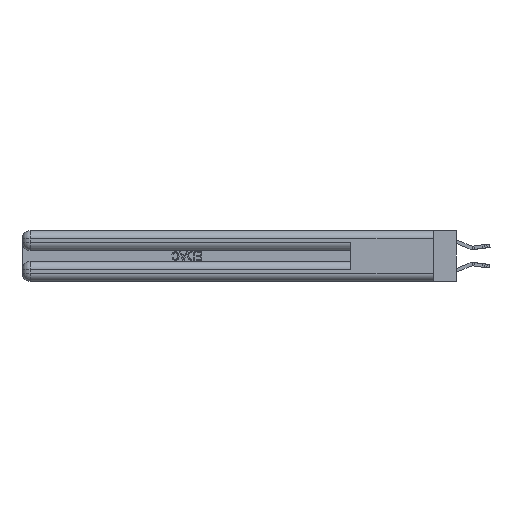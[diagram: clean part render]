
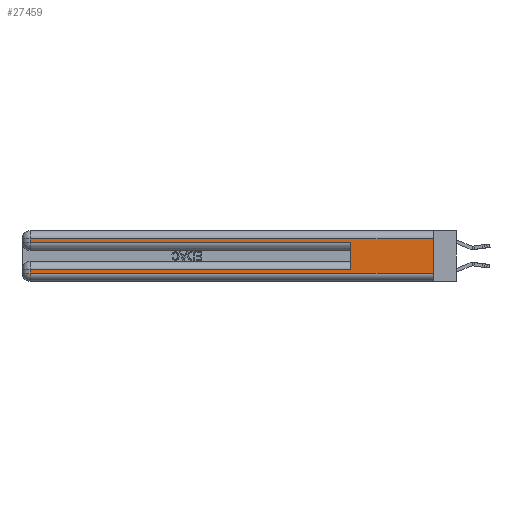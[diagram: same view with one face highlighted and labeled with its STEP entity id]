
A CAD part, left-side view. The second image highlights one B-rep face of the part: STEP entity #27459.
In plain terms, the highlighted planar face has unit normal (-1, 0, 0).
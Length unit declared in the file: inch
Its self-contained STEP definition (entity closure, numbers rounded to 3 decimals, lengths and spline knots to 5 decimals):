
#120 = CARTESIAN_POINT ( 'NONE',  ( 0., 0., 0.31 ) ) ;
#1399 = ORIENTED_EDGE ( 'NONE', *, *, #13065, .F. ) ;
#3127 = ORIENTED_EDGE ( 'NONE', *, *, #30233, .T. ) ;
#3662 = CARTESIAN_POINT ( 'NONE',  ( 0., 2.94, 0.06 ) ) ;
#4839 = VECTOR ( 'NONE', #20133, 39.37008 ) ;
#5645 = DIRECTION ( 'NONE',  ( 1., 0., 0. ) ) ;
#6903 = VERTEX_POINT ( 'NONE', #29737 ) ;
#7771 = LINE ( 'NONE', #35085, #21721 ) ;
#8116 = LINE ( 'NONE', #36131, #30444 ) ;
#8566 = VECTOR ( 'NONE', #29081, 39.37008 ) ;
#8810 = LINE ( 'NONE', #13222, #31150 ) ;
#10208 = EDGE_CURVE ( 'NONE', #28168, #25118, #15993, .T. ) ;
#10483 = EDGE_CURVE ( 'NONE', #6903, #19917, #8116, .T. ) ;
#11653 = EDGE_CURVE ( 'NONE', #18416, #22602, #7771, .T. ) ;
#11715 = CARTESIAN_POINT ( 'NONE',  ( 0., 0., 0.06 ) ) ;
#11868 = ORIENTED_EDGE ( 'NONE', *, *, #10208, .F. ) ;
#11930 = CARTESIAN_POINT ( 'NONE',  ( 0., 2.94, 0.085 ) ) ;
#13065 = EDGE_CURVE ( 'NONE', #18416, #27856, #30847, .T. ) ;
#13222 = CARTESIAN_POINT ( 'NONE',  ( 0., 0., 0.31 ) ) ;
#13622 = ORIENTED_EDGE ( 'NONE', *, *, #15693, .T. ) ;
#14135 = DIRECTION ( 'NONE',  ( 0., -1., 0. ) ) ;
#14506 = ORIENTED_EDGE ( 'NONE', *, *, #24311, .T. ) ;
#15693 = EDGE_CURVE ( 'NONE', #28168, #6903, #8810, .T. ) ;
#15993 = LINE ( 'NONE', #26271, #8566 ) ;
#16026 = EDGE_LOOP ( 'NONE', ( #11868, #13622, #28511, #14506, #1399, #23707, #24590, #3127 ) ) ;
#16344 = LINE ( 'NONE', #28599, #22025 ) ;
#16733 = PLANE ( 'NONE',  #16895 ) ;
#16895 = AXIS2_PLACEMENT_3D ( 'NONE', #19566, #5645, #25209 ) ;
#18416 = VERTEX_POINT ( 'NONE', #29125 ) ;
#18808 = LINE ( 'NONE', #11715, #4839 ) ;
#19365 = DIRECTION ( 'NONE',  ( 0., 0., -1. ) ) ;
#19566 = CARTESIAN_POINT ( 'NONE',  ( 0., 0., 0.37 ) ) ;
#19917 = VERTEX_POINT ( 'NONE', #22398 ) ;
#20133 = DIRECTION ( 'NONE',  ( 0., -1., 0. ) ) ;
#20135 = DIRECTION ( 'NONE',  ( 0., 0., -1. ) ) ;
#21721 = VECTOR ( 'NONE', #23969, 39.37008 ) ;
#22025 = VECTOR ( 'NONE', #20135, 39.37008 ) ;
#22398 = CARTESIAN_POINT ( 'NONE',  ( 0., 2.94, 0.285 ) ) ;
#22486 = VECTOR ( 'NONE', #28692, 39.37008 ) ;
#22602 = VERTEX_POINT ( 'NONE', #11930 ) ;
#23707 = ORIENTED_EDGE ( 'NONE', *, *, #11653, .T. ) ;
#23969 = DIRECTION ( 'NONE',  ( 0., 1., 0. ) ) ;
#24311 = EDGE_CURVE ( 'NONE', #19917, #27856, #27111, .T. ) ;
#24590 = ORIENTED_EDGE ( 'NONE', *, *, #34858, .T. ) ;
#25118 = VERTEX_POINT ( 'NONE', #28905 ) ;
#25209 = DIRECTION ( 'NONE',  ( 0., 0., -1. ) ) ;
#26271 = CARTESIAN_POINT ( 'NONE',  ( 0., 0., 0.37 ) ) ;
#26449 = FACE_OUTER_BOUND ( 'NONE', #16026, .T. ) ;
#27111 = LINE ( 'NONE', #28088, #34535 ) ;
#27459 = ADVANCED_FACE ( 'NONE', ( #26449 ), #16733, .F. ) ;
#27657 = VERTEX_POINT ( 'NONE', #3662 ) ;
#27856 = VERTEX_POINT ( 'NONE', #29623 ) ;
#28088 = CARTESIAN_POINT ( 'NONE',  ( 0., 0., 0.285 ) ) ;
#28168 = VERTEX_POINT ( 'NONE', #120 ) ;
#28511 = ORIENTED_EDGE ( 'NONE', *, *, #10483, .T. ) ;
#28599 = CARTESIAN_POINT ( 'NONE',  ( 0., 2.94, 0.37 ) ) ;
#28692 = DIRECTION ( 'NONE',  ( 0., 0., 1. ) ) ;
#28905 = CARTESIAN_POINT ( 'NONE',  ( 0., 0., 0.06 ) ) ;
#29081 = DIRECTION ( 'NONE',  ( 0., 0., -1. ) ) ;
#29125 = CARTESIAN_POINT ( 'NONE',  ( 0., 0.6, 0.085 ) ) ;
#29623 = CARTESIAN_POINT ( 'NONE',  ( 0., 0.6, 0.285 ) ) ;
#29737 = CARTESIAN_POINT ( 'NONE',  ( 0., 2.94, 0.31 ) ) ;
#30003 = DIRECTION ( 'NONE',  ( 0., 1., 0. ) ) ;
#30233 = EDGE_CURVE ( 'NONE', #27657, #25118, #18808, .T. ) ;
#30444 = VECTOR ( 'NONE', #19365, 39.37008 ) ;
#30847 = LINE ( 'NONE', #34299, #22486 ) ;
#31150 = VECTOR ( 'NONE', #30003, 39.37008 ) ;
#34299 = CARTESIAN_POINT ( 'NONE',  ( 0., 0.6, 0.145 ) ) ;
#34535 = VECTOR ( 'NONE', #14135, 39.37008 ) ;
#34858 = EDGE_CURVE ( 'NONE', #22602, #27657, #16344, .T. ) ;
#35085 = CARTESIAN_POINT ( 'NONE',  ( 0., 0., 0.085 ) ) ;
#36131 = CARTESIAN_POINT ( 'NONE',  ( 0., 2.94, 0.37 ) ) ;
